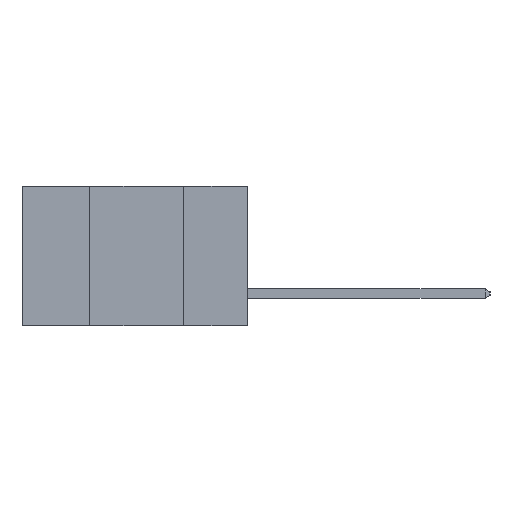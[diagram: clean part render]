
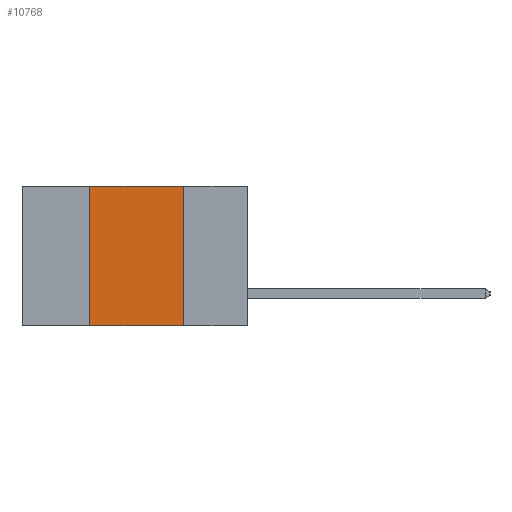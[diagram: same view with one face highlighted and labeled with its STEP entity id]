
A CAD part, left-side view. The second image highlights one B-rep face of the part: STEP entity #10768.
In plain terms, the highlighted planar face has unit normal (-1, 0, 0).
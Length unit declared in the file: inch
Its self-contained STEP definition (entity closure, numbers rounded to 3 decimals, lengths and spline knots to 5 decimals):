
#458 = EDGE_CURVE ( 'NONE', #962, #11819, #10792, .T. ) ;
#556 = VERTEX_POINT ( 'NONE', #5357 ) ;
#614 = VECTOR ( 'NONE', #11596, 39.37008 ) ;
#835 = PLANE ( 'NONE',  #7714 ) ;
#962 = VERTEX_POINT ( 'NONE', #10438 ) ;
#1530 = LINE ( 'NONE', #11877, #614 ) ;
#1659 = VERTEX_POINT ( 'NONE', #8301 ) ;
#1798 = DIRECTION ( 'NONE',  ( 0., 0., -1. ) ) ;
#2636 = EDGE_CURVE ( 'NONE', #1659, #11819, #1530, .T. ) ;
#3260 = LINE ( 'NONE', #9502, #7439 ) ;
#3860 = DIRECTION ( 'NONE',  ( 0., -1., 0. ) ) ;
#4223 = LINE ( 'NONE', #12078, #6463 ) ;
#4684 = ORIENTED_EDGE ( 'NONE', *, *, #458, .F. ) ;
#4690 = CARTESIAN_POINT ( 'NONE',  ( 0., 0.6, 0. ) ) ;
#4694 = ORIENTED_EDGE ( 'NONE', *, *, #9578, .F. ) ;
#4727 = ORIENTED_EDGE ( 'NONE', *, *, #7768, .F. ) ;
#4737 = ORIENTED_EDGE ( 'NONE', *, *, #2636, .T. ) ;
#4949 = FACE_OUTER_BOUND ( 'NONE', #9810, .T. ) ;
#5357 = CARTESIAN_POINT ( 'NONE',  ( 0., 0.42, 0. ) ) ;
#6463 = VECTOR ( 'NONE', #9411, 39.37008 ) ;
#7227 = CARTESIAN_POINT ( 'NONE',  ( 0., 0.17, -0.37 ) ) ;
#7439 = VECTOR ( 'NONE', #3860, 39.37008 ) ;
#7531 = DIRECTION ( 'NONE',  ( 1., 0., 0. ) ) ;
#7714 = AXIS2_PLACEMENT_3D ( 'NONE', #4690, #7531, #1798 ) ;
#7768 = EDGE_CURVE ( 'NONE', #1659, #556, #4223, .T. ) ;
#8301 = CARTESIAN_POINT ( 'NONE',  ( 0., 0.42, -0.37 ) ) ;
#8424 = VECTOR ( 'NONE', #9656, 39.37008 ) ;
#9204 = CARTESIAN_POINT ( 'NONE',  ( 0., 0.17, -0.37 ) ) ;
#9411 = DIRECTION ( 'NONE',  ( 0., 0., 1. ) ) ;
#9502 = CARTESIAN_POINT ( 'NONE',  ( 0., 0.6, 0. ) ) ;
#9578 = EDGE_CURVE ( 'NONE', #556, #962, #3260, .T. ) ;
#9656 = DIRECTION ( 'NONE',  ( 0., 0., -1. ) ) ;
#9810 = EDGE_LOOP ( 'NONE', ( #4684, #4694, #4727, #4737 ) ) ;
#10438 = CARTESIAN_POINT ( 'NONE',  ( 0., 0.17, 0. ) ) ;
#10768 = ADVANCED_FACE ( 'NONE', ( #4949 ), #835, .F. ) ;
#10792 = LINE ( 'NONE', #9204, #8424 ) ;
#11596 = DIRECTION ( 'NONE',  ( 0., -1., 0. ) ) ;
#11819 = VERTEX_POINT ( 'NONE', #7227 ) ;
#11877 = CARTESIAN_POINT ( 'NONE',  ( 0., 0.6, -0.37 ) ) ;
#12078 = CARTESIAN_POINT ( 'NONE',  ( 0., 0.42, -0.37 ) ) ;
